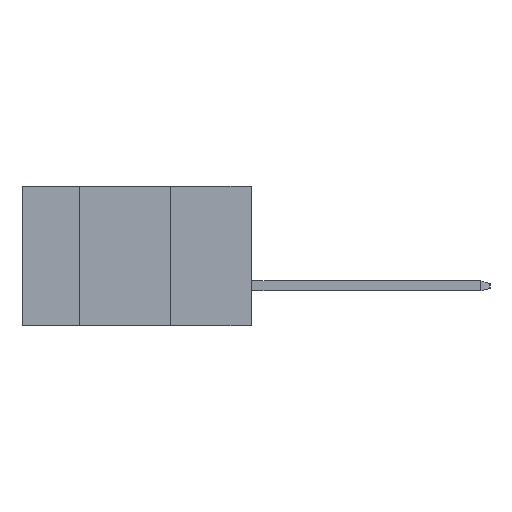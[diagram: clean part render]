
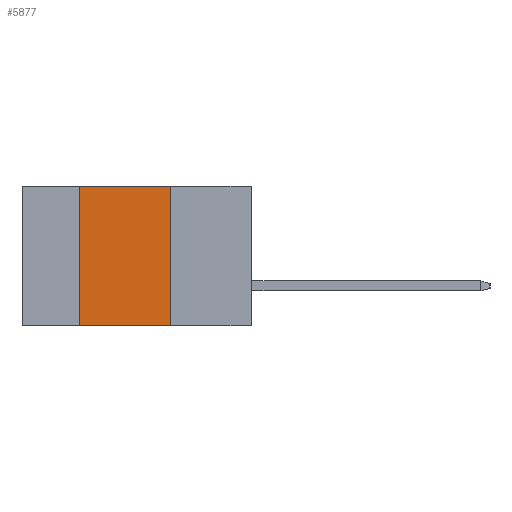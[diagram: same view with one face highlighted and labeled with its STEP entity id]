
A CAD part, left-side view. The second image highlights one B-rep face of the part: STEP entity #5877.
In plain terms, the highlighted planar face has unit normal (-1, 0, 0).
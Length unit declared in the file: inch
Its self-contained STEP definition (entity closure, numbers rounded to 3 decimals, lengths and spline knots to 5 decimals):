
#117 = VERTEX_POINT ( 'NONE', #3802 ) ;
#756 = EDGE_CURVE ( 'NONE', #2997, #4486, #1067, .T. ) ;
#1067 = LINE ( 'NONE', #7005, #6259 ) ;
#1217 = CARTESIAN_POINT ( 'NONE',  ( 0., 0.54, -0.437 ) ) ;
#1608 = ORIENTED_EDGE ( 'NONE', *, *, #756, .F. ) ;
#1719 = EDGE_CURVE ( 'NONE', #117, #2997, #8662, .T. ) ;
#1939 = LINE ( 'NONE', #1217, #4729 ) ;
#2285 = VERTEX_POINT ( 'NONE', #6521 ) ;
#2734 = CARTESIAN_POINT ( 'NONE',  ( 0., 0.72, 0. ) ) ;
#2997 = VERTEX_POINT ( 'NONE', #7863 ) ;
#3263 = DIRECTION ( 'NONE',  ( 0., 0., -1. ) ) ;
#3411 = CARTESIAN_POINT ( 'NONE',  ( 0., 0.72, -0.437 ) ) ;
#3588 = DIRECTION ( 'NONE',  ( 0., 0., -1. ) ) ;
#3680 = CARTESIAN_POINT ( 'NONE',  ( 0., 0.72, 0. ) ) ;
#3802 = CARTESIAN_POINT ( 'NONE',  ( 0., 0.54, 0. ) ) ;
#4180 = DIRECTION ( 'NONE',  ( 0., 0., 1. ) ) ;
#4486 = VERTEX_POINT ( 'NONE', #6117 ) ;
#4619 = ORIENTED_EDGE ( 'NONE', *, *, #1719, .F. ) ;
#4729 = VECTOR ( 'NONE', #4180, 39.37008 ) ;
#4741 = DIRECTION ( 'NONE',  ( 0., -1., 0. ) ) ;
#4784 = LINE ( 'NONE', #3411, #7815 ) ;
#5364 = ORIENTED_EDGE ( 'NONE', *, *, #8233, .T. ) ;
#5375 = AXIS2_PLACEMENT_3D ( 'NONE', #3680, #6659, #3588 ) ;
#5724 = DIRECTION ( 'NONE',  ( 0., -1., 0. ) ) ;
#5877 = ADVANCED_FACE ( 'NONE', ( #8792 ), #8111, .F. ) ;
#6117 = CARTESIAN_POINT ( 'NONE',  ( 0., 0.254, -0.437 ) ) ;
#6124 = VECTOR ( 'NONE', #5724, 39.37008 ) ;
#6259 = VECTOR ( 'NONE', #3263, 39.37008 ) ;
#6521 = CARTESIAN_POINT ( 'NONE',  ( 0., 0.54, -0.437 ) ) ;
#6659 = DIRECTION ( 'NONE',  ( 1., 0., 0. ) ) ;
#7005 = CARTESIAN_POINT ( 'NONE',  ( 0., 0.254, -0.437 ) ) ;
#7611 = ORIENTED_EDGE ( 'NONE', *, *, #8896, .F. ) ;
#7815 = VECTOR ( 'NONE', #4741, 39.37008 ) ;
#7863 = CARTESIAN_POINT ( 'NONE',  ( 0., 0.254, 0. ) ) ;
#8111 = PLANE ( 'NONE',  #5375 ) ;
#8183 = EDGE_LOOP ( 'NONE', ( #1608, #4619, #7611, #5364 ) ) ;
#8233 = EDGE_CURVE ( 'NONE', #2285, #4486, #4784, .T. ) ;
#8662 = LINE ( 'NONE', #2734, #6124 ) ;
#8792 = FACE_OUTER_BOUND ( 'NONE', #8183, .T. ) ;
#8896 = EDGE_CURVE ( 'NONE', #2285, #117, #1939, .T. ) ;
